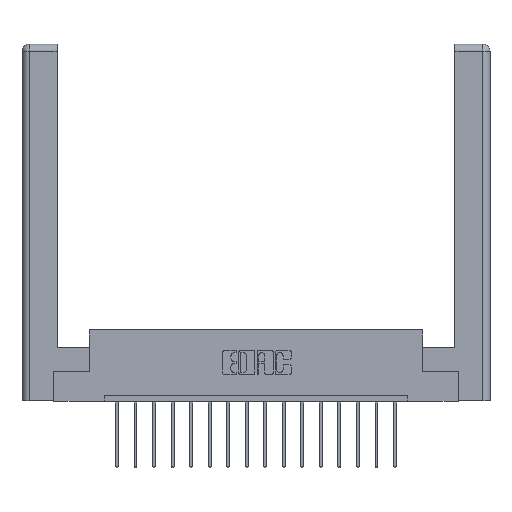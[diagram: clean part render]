
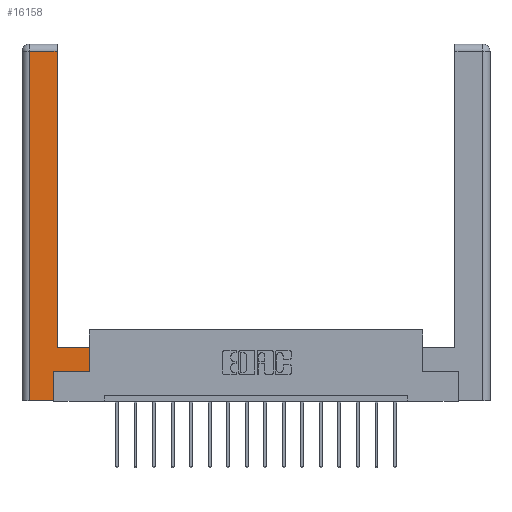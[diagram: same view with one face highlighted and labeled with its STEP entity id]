
A CAD part, top view. The second image highlights one B-rep face of the part: STEP entity #16158.
In plain terms, the highlighted planar face has unit normal (0, 0, 1).
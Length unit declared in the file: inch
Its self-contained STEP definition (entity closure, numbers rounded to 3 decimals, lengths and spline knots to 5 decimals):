
#181 = VECTOR ( 'NONE', #9413, 39.37008 ) ;
#466 = ORIENTED_EDGE ( 'NONE', *, *, #8670, .T. ) ;
#652 = EDGE_CURVE ( 'NONE', #11999, #14201, #4040, .T. ) ;
#959 = VERTEX_POINT ( 'NONE', #10993 ) ;
#1110 = CARTESIAN_POINT ( 'NONE',  ( 0.265, 0., 0. ) ) ;
#1194 = CARTESIAN_POINT ( 'NONE',  ( 0.565, 0.245, 0. ) ) ;
#1258 = ORIENTED_EDGE ( 'NONE', *, *, #9834, .T. ) ;
#1281 = VERTEX_POINT ( 'NONE', #15799 ) ;
#1526 = CARTESIAN_POINT ( 'NONE',  ( 0.565, 0.45, 0. ) ) ;
#1547 = EDGE_CURVE ( 'NONE', #959, #11999, #11363, .T. ) ;
#1939 = CARTESIAN_POINT ( 'NONE',  ( 0.0615, 0., 0. ) ) ;
#2533 = DIRECTION ( 'NONE',  ( 0., 1., 0. ) ) ;
#2758 = VECTOR ( 'NONE', #16306, 39.37008 ) ;
#3231 = EDGE_CURVE ( 'NONE', #10878, #1281, #12260, .T. ) ;
#3278 = ORIENTED_EDGE ( 'NONE', *, *, #14626, .T. ) ;
#3403 = LINE ( 'NONE', #9358, #2758 ) ;
#3404 = VECTOR ( 'NONE', #5793, 39.37008 ) ;
#4040 = LINE ( 'NONE', #14645, #6005 ) ;
#4837 = CARTESIAN_POINT ( 'NONE',  ( 0.0615, 2.94, 0. ) ) ;
#5534 = VERTEX_POINT ( 'NONE', #7962 ) ;
#5708 = PLANE ( 'NONE',  #6066 ) ;
#5793 = DIRECTION ( 'NONE',  ( 0., 1., 0. ) ) ;
#6005 = VECTOR ( 'NONE', #14190, 39.37008 ) ;
#6066 = AXIS2_PLACEMENT_3D ( 'NONE', #16555, #15338, #6904 ) ;
#6205 = LINE ( 'NONE', #9864, #3404 ) ;
#6477 = LINE ( 'NONE', #4837, #181 ) ;
#6904 = DIRECTION ( 'NONE',  ( -1., 0., 0. ) ) ;
#7715 = LINE ( 'NONE', #14502, #15046 ) ;
#7962 = CARTESIAN_POINT ( 'NONE',  ( 0.295, 0.45, 0. ) ) ;
#8487 = EDGE_CURVE ( 'NONE', #1281, #17488, #7715, .T. ) ;
#8529 = ORIENTED_EDGE ( 'NONE', *, *, #1547, .T. ) ;
#8670 = EDGE_CURVE ( 'NONE', #14201, #5534, #3403, .T. ) ;
#9358 = CARTESIAN_POINT ( 'NONE',  ( 0.295, 0.45, 0. ) ) ;
#9413 = DIRECTION ( 'NONE',  ( -1., 0., 0. ) ) ;
#9834 = EDGE_CURVE ( 'NONE', #5534, #17173, #12628, .T. ) ;
#9864 = CARTESIAN_POINT ( 'NONE',  ( 0.265, 0.245, 0. ) ) ;
#10193 = DIRECTION ( 'NONE',  ( 0., -1., 0. ) ) ;
#10437 = DIRECTION ( 'NONE',  ( 1., 0., 0. ) ) ;
#10878 = VERTEX_POINT ( 'NONE', #14302 ) ;
#10993 = CARTESIAN_POINT ( 'NONE',  ( 0.265, 0.245, 0. ) ) ;
#11363 = LINE ( 'NONE', #12629, #12851 ) ;
#11926 = EDGE_LOOP ( 'NONE', ( #1258, #3278, #12257, #12978, #17242, #8529, #13322, #466 ) ) ;
#11999 = VERTEX_POINT ( 'NONE', #1194 ) ;
#12257 = ORIENTED_EDGE ( 'NONE', *, *, #3231, .T. ) ;
#12260 = LINE ( 'NONE', #1939, #14230 ) ;
#12628 = LINE ( 'NONE', #17728, #14160 ) ;
#12629 = CARTESIAN_POINT ( 'NONE',  ( 0.565, 0.245, 0. ) ) ;
#12851 = VECTOR ( 'NONE', #15345, 39.37008 ) ;
#12978 = ORIENTED_EDGE ( 'NONE', *, *, #8487, .T. ) ;
#13322 = ORIENTED_EDGE ( 'NONE', *, *, #652, .T. ) ;
#14160 = VECTOR ( 'NONE', #2533, 39.37008 ) ;
#14190 = DIRECTION ( 'NONE',  ( 0., 1., 0. ) ) ;
#14201 = VERTEX_POINT ( 'NONE', #1526 ) ;
#14230 = VECTOR ( 'NONE', #10193, 39.37008 ) ;
#14302 = CARTESIAN_POINT ( 'NONE',  ( 0.0615, 2.94, 0. ) ) ;
#14502 = CARTESIAN_POINT ( 'NONE',  ( 0.265, 0., 0. ) ) ;
#14626 = EDGE_CURVE ( 'NONE', #17173, #10878, #6477, .T. ) ;
#14645 = CARTESIAN_POINT ( 'NONE',  ( 0.565, 0.45, 0. ) ) ;
#15046 = VECTOR ( 'NONE', #10437, 39.37008 ) ;
#15338 = DIRECTION ( 'NONE',  ( 0., 0., -1. ) ) ;
#15345 = DIRECTION ( 'NONE',  ( 1., 0., 0. ) ) ;
#15687 = FACE_OUTER_BOUND ( 'NONE', #11926, .T. ) ;
#15772 = EDGE_CURVE ( 'NONE', #17488, #959, #6205, .T. ) ;
#15799 = CARTESIAN_POINT ( 'NONE',  ( 0.0615, 0., 0. ) ) ;
#16158 = ADVANCED_FACE ( 'NONE', ( #15687 ), #5708, .F. ) ;
#16306 = DIRECTION ( 'NONE',  ( -1., 0., 0. ) ) ;
#16555 = CARTESIAN_POINT ( 'NONE',  ( 0., 0., 0. ) ) ;
#17173 = VERTEX_POINT ( 'NONE', #17471 ) ;
#17242 = ORIENTED_EDGE ( 'NONE', *, *, #15772, .T. ) ;
#17471 = CARTESIAN_POINT ( 'NONE',  ( 0.295, 2.94, 0. ) ) ;
#17488 = VERTEX_POINT ( 'NONE', #1110 ) ;
#17728 = CARTESIAN_POINT ( 'NONE',  ( 0.295, 3., 0. ) ) ;
